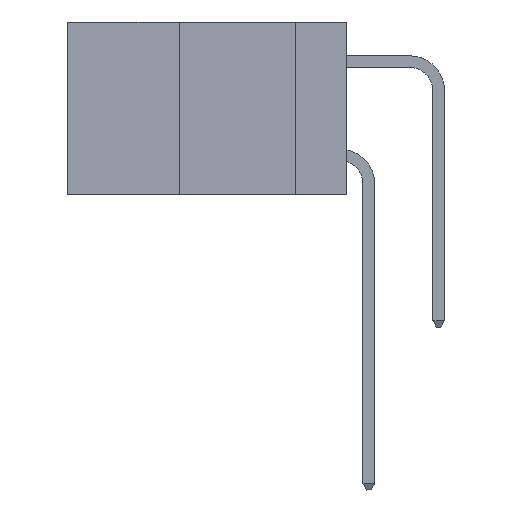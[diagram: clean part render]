
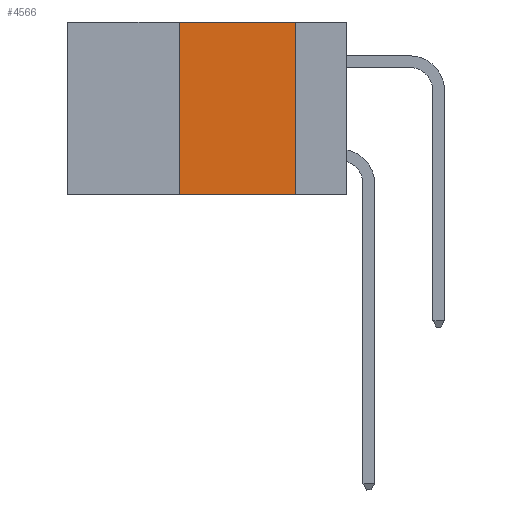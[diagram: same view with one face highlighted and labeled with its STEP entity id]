
A CAD part, left-side view. The second image highlights one B-rep face of the part: STEP entity #4566.
In plain terms, the highlighted planar face has unit normal (-1, 0, 0).
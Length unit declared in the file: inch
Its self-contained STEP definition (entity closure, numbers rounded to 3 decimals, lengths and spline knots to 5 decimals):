
#229 = VERTEX_POINT ( 'NONE', #4030 ) ;
#537 = EDGE_LOOP ( 'NONE', ( #2981, #18633, #21371, #3389 ) ) ;
#822 = LINE ( 'NONE', #5256, #2755 ) ;
#961 = VECTOR ( 'NONE', #8623, 39.37008 ) ;
#1301 = DIRECTION ( 'NONE',  ( 0., 0., 1. ) ) ;
#1467 = CARTESIAN_POINT ( 'NONE',  ( 0., 0.6, -0.37 ) ) ;
#2755 = VECTOR ( 'NONE', #10303, 39.37008 ) ;
#2981 = ORIENTED_EDGE ( 'NONE', *, *, #18054, .F. ) ;
#3104 = CARTESIAN_POINT ( 'NONE',  ( 0., 0.11, -0.37 ) ) ;
#3389 = ORIENTED_EDGE ( 'NONE', *, *, #15789, .T. ) ;
#4030 = CARTESIAN_POINT ( 'NONE',  ( 0., 0.36, 0. ) ) ;
#4566 = ADVANCED_FACE ( 'NONE', ( #6028 ), #18900, .F. ) ;
#5256 = CARTESIAN_POINT ( 'NONE',  ( 0., 0.11, 0. ) ) ;
#6028 = FACE_OUTER_BOUND ( 'NONE', #537, .T. ) ;
#6181 = AXIS2_PLACEMENT_3D ( 'NONE', #11855, #13516, #18741 ) ;
#6273 = VERTEX_POINT ( 'NONE', #3104 ) ;
#7167 = VERTEX_POINT ( 'NONE', #19891 ) ;
#8405 = EDGE_CURVE ( 'NONE', #7167, #229, #17857, .T. ) ;
#8623 = DIRECTION ( 'NONE',  ( 0., -1., 0. ) ) ;
#10050 = EDGE_CURVE ( 'NONE', #229, #17504, #18023, .T. ) ;
#10303 = DIRECTION ( 'NONE',  ( 0., 0., -1. ) ) ;
#11855 = CARTESIAN_POINT ( 'NONE',  ( 0., 0.6, 0. ) ) ;
#13516 = DIRECTION ( 'NONE',  ( 1., 0., 0. ) ) ;
#15144 = CARTESIAN_POINT ( 'NONE',  ( 0., 0.11, 0. ) ) ;
#15789 = EDGE_CURVE ( 'NONE', #7167, #6273, #16258, .T. ) ;
#16258 = LINE ( 'NONE', #1467, #961 ) ;
#16349 = CARTESIAN_POINT ( 'NONE',  ( 0., 0.6, 0. ) ) ;
#17504 = VERTEX_POINT ( 'NONE', #15144 ) ;
#17857 = LINE ( 'NONE', #20788, #21431 ) ;
#18023 = LINE ( 'NONE', #16349, #20793 ) ;
#18054 = EDGE_CURVE ( 'NONE', #17504, #6273, #822, .T. ) ;
#18633 = ORIENTED_EDGE ( 'NONE', *, *, #10050, .F. ) ;
#18741 = DIRECTION ( 'NONE',  ( 0., 0., -1. ) ) ;
#18900 = PLANE ( 'NONE',  #6181 ) ;
#19891 = CARTESIAN_POINT ( 'NONE',  ( 0., 0.36, -0.37 ) ) ;
#20788 = CARTESIAN_POINT ( 'NONE',  ( 0., 0.36, 0. ) ) ;
#20793 = VECTOR ( 'NONE', #21739, 39.37008 ) ;
#21371 = ORIENTED_EDGE ( 'NONE', *, *, #8405, .F. ) ;
#21431 = VECTOR ( 'NONE', #1301, 39.37008 ) ;
#21739 = DIRECTION ( 'NONE',  ( 0., -1., 0. ) ) ;
